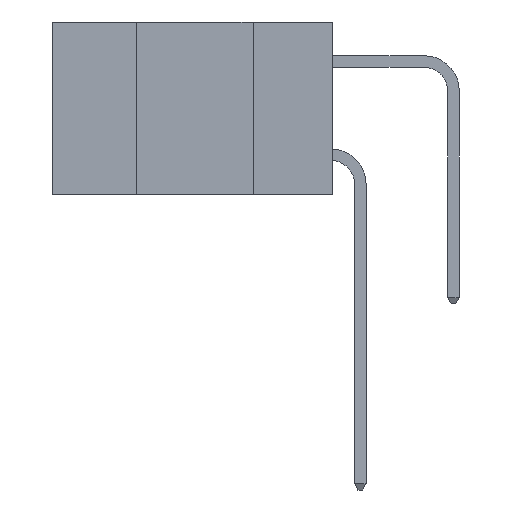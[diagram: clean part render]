
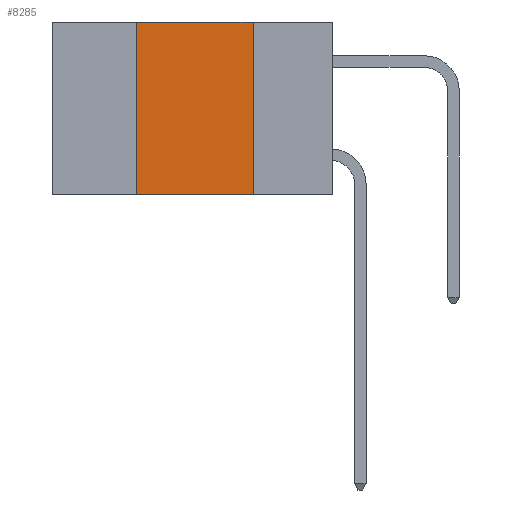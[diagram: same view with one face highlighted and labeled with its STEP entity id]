
A CAD part, left-side view. The second image highlights one B-rep face of the part: STEP entity #8285.
In plain terms, the highlighted planar face has unit normal (-1, 0, 0).
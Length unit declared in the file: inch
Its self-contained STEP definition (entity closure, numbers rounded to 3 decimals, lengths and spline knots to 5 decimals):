
#655 = PLANE ( 'NONE',  #8937 ) ;
#1257 = VECTOR ( 'NONE', #5553, 39.37008 ) ;
#2123 = DIRECTION ( 'NONE',  ( 1., 0., 0. ) ) ;
#2785 = CARTESIAN_POINT ( 'NONE',  ( 0., 0.42, -0.37 ) ) ;
#2991 = LINE ( 'NONE', #3235, #16812 ) ;
#3235 = CARTESIAN_POINT ( 'NONE',  ( 0., 0.6, -0.37 ) ) ;
#3298 = ORIENTED_EDGE ( 'NONE', *, *, #13606, .F. ) ;
#3636 = VERTEX_POINT ( 'NONE', #13247 ) ;
#4416 = EDGE_CURVE ( 'NONE', #15611, #4999, #16192, .T. ) ;
#4433 = CARTESIAN_POINT ( 'NONE',  ( 0., 0.17, 0. ) ) ;
#4558 = ORIENTED_EDGE ( 'NONE', *, *, #16393, .T. ) ;
#4860 = EDGE_LOOP ( 'NONE', ( #7198, #6038, #3298, #4558 ) ) ;
#4999 = VERTEX_POINT ( 'NONE', #7423 ) ;
#5140 = VECTOR ( 'NONE', #12594, 39.37008 ) ;
#5553 = DIRECTION ( 'NONE',  ( 0., 0., 1. ) ) ;
#6038 = ORIENTED_EDGE ( 'NONE', *, *, #12640, .F. ) ;
#6620 = VERTEX_POINT ( 'NONE', #2785 ) ;
#7198 = ORIENTED_EDGE ( 'NONE', *, *, #4416, .F. ) ;
#7299 = DIRECTION ( 'NONE',  ( 0., -1., 0. ) ) ;
#7423 = CARTESIAN_POINT ( 'NONE',  ( 0., 0.17, -0.37 ) ) ;
#8285 = ADVANCED_FACE ( 'NONE', ( #15622 ), #655, .F. ) ;
#8937 = AXIS2_PLACEMENT_3D ( 'NONE', #10425, #2123, #11773 ) ;
#10425 = CARTESIAN_POINT ( 'NONE',  ( 0., 0.6, 0. ) ) ;
#11773 = DIRECTION ( 'NONE',  ( 0., 0., -1. ) ) ;
#12437 = CARTESIAN_POINT ( 'NONE',  ( 0., 0.42, -0.37 ) ) ;
#12594 = DIRECTION ( 'NONE',  ( 0., 0., -1. ) ) ;
#12629 = CARTESIAN_POINT ( 'NONE',  ( 0., 0.17, -0.37 ) ) ;
#12640 = EDGE_CURVE ( 'NONE', #3636, #15611, #15477, .T. ) ;
#13247 = CARTESIAN_POINT ( 'NONE',  ( 0., 0.42, 0. ) ) ;
#13382 = DIRECTION ( 'NONE',  ( 0., -1., 0. ) ) ;
#13606 = EDGE_CURVE ( 'NONE', #6620, #3636, #15895, .T. ) ;
#15477 = LINE ( 'NONE', #16176, #17780 ) ;
#15611 = VERTEX_POINT ( 'NONE', #4433 ) ;
#15622 = FACE_OUTER_BOUND ( 'NONE', #4860, .T. ) ;
#15895 = LINE ( 'NONE', #12437, #1257 ) ;
#16176 = CARTESIAN_POINT ( 'NONE',  ( 0., 0.6, 0. ) ) ;
#16192 = LINE ( 'NONE', #12629, #5140 ) ;
#16393 = EDGE_CURVE ( 'NONE', #6620, #4999, #2991, .T. ) ;
#16812 = VECTOR ( 'NONE', #7299, 39.37008 ) ;
#17780 = VECTOR ( 'NONE', #13382, 39.37008 ) ;
